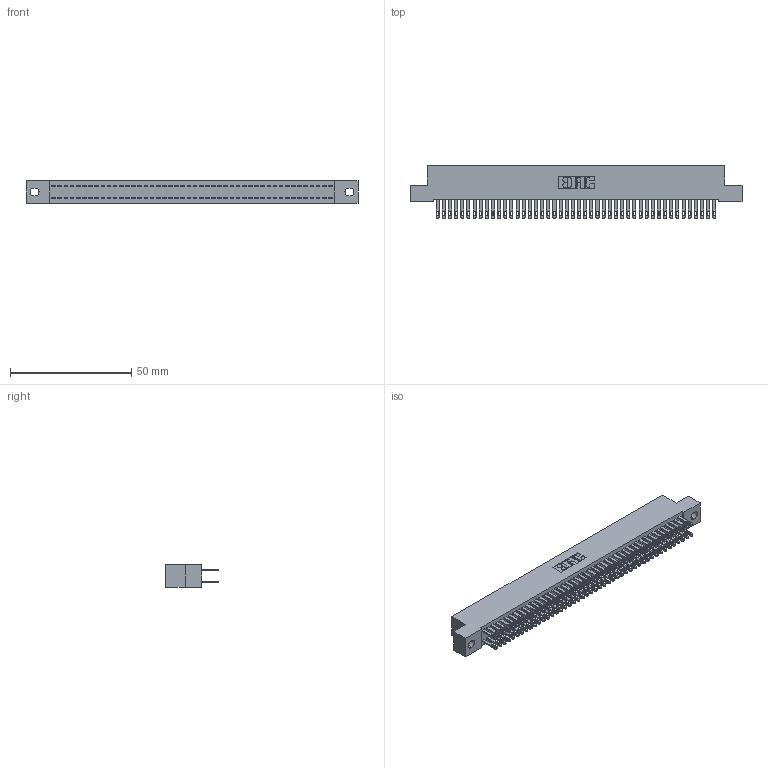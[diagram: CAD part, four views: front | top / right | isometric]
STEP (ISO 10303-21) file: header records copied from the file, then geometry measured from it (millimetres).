
FILE_DESCRIPTION (( 'STEP AP203' ), '1' );
FILE_NAME ('892-092-500-202.STEP', '2020-09-21T20:49:49', ( '' ), ( '' ), 'SwSTEP 2.0', 'SolidWorks 2020', '' );
FILE_SCHEMA (( 'CONFIG_CONTROL_DESIGN' ));
Length unit declared in the file: inch
Products named in the file (3): 842 Part_.128 Slot; 892-092-500-202; 345-292-001_345-293-100
Assembly tree (93 placements, depth 2):
  892-092-500-202
    842 Part_.128 Slot
    345-292-001_345-293-100  x92
Bounding box: 137.16 x 21.85 x 9.4 mm (x, y, z)
Volume: 12571.7 mm3; surface area: 21202.5 mm2
Topology: 93 solids, 93 shells, 4530 faces, 13835 edges, 9222 vertices
Faces by surface type: plane 2830, cylinder 1700
Entity records: 29009 total; most frequent: CARTESIAN_POINT 4802, ORIENTED_EDGE 4738, DIRECTION 4097, EDGE_CURVE 2369, VECTOR 2237, LINE 2237, VERTEX_POINT 1578, AXIS2_PLACEMENT_3D 930
